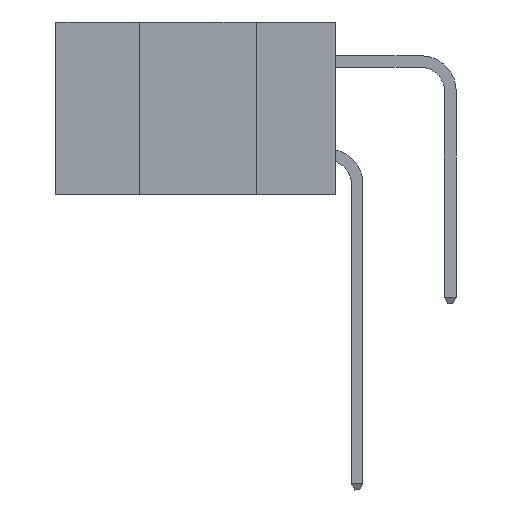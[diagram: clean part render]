
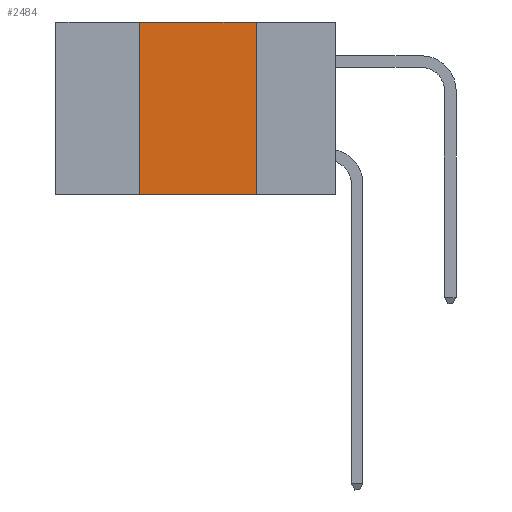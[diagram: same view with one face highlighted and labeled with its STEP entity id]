
A CAD part, left-side view. The second image highlights one B-rep face of the part: STEP entity #2484.
In plain terms, the highlighted planar face has unit normal (-1, 0, 0).
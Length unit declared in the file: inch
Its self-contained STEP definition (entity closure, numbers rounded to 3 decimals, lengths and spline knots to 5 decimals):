
#271 = ORIENTED_EDGE ( 'NONE', *, *, #18423, .F. ) ;
#292 = VECTOR ( 'NONE', #7516, 39.37008 ) ;
#970 = AXIS2_PLACEMENT_3D ( 'NONE', #7529, #13797, #14247 ) ;
#1434 = LINE ( 'NONE', #8473, #26179 ) ;
#1643 = VERTEX_POINT ( 'NONE', #16761 ) ;
#2484 = ADVANCED_FACE ( 'NONE', ( #3486 ), #12057, .F. ) ;
#2525 = VECTOR ( 'NONE', #13872, 39.37008 ) ;
#2787 = CARTESIAN_POINT ( 'NONE',  ( 0., 0.42, -0.37 ) ) ;
#3486 = FACE_OUTER_BOUND ( 'NONE', #3896, .T. ) ;
#3793 = CARTESIAN_POINT ( 'NONE',  ( 0., 0.42, 0. ) ) ;
#3896 = EDGE_LOOP ( 'NONE', ( #23246, #271, #9026, #25586 ) ) ;
#6519 = LINE ( 'NONE', #3793, #11027 ) ;
#6774 = LINE ( 'NONE', #26306, #2525 ) ;
#7516 = DIRECTION ( 'NONE',  ( 0., -1., 0. ) ) ;
#7529 = CARTESIAN_POINT ( 'NONE',  ( 0., 0.6, 0. ) ) ;
#8417 = EDGE_CURVE ( 'NONE', #19377, #11493, #6774, .T. ) ;
#8473 = CARTESIAN_POINT ( 'NONE',  ( 0., 0.17, 0. ) ) ;
#9026 = ORIENTED_EDGE ( 'NONE', *, *, #18155, .F. ) ;
#11027 = VECTOR ( 'NONE', #16083, 39.37008 ) ;
#11493 = VERTEX_POINT ( 'NONE', #21576 ) ;
#12057 = PLANE ( 'NONE',  #970 ) ;
#13797 = DIRECTION ( 'NONE',  ( 1., 0., 0. ) ) ;
#13872 = DIRECTION ( 'NONE',  ( 0., -1., 0. ) ) ;
#14247 = DIRECTION ( 'NONE',  ( 0., 0., -1. ) ) ;
#16083 = DIRECTION ( 'NONE',  ( 0., 0., 1. ) ) ;
#16761 = CARTESIAN_POINT ( 'NONE',  ( 0., 0.17, 0. ) ) ;
#17349 = EDGE_CURVE ( 'NONE', #1643, #11493, #1434, .T. ) ;
#18155 = EDGE_CURVE ( 'NONE', #19377, #22650, #6519, .T. ) ;
#18423 = EDGE_CURVE ( 'NONE', #22650, #1643, #23109, .T. ) ;
#18897 = CARTESIAN_POINT ( 'NONE',  ( 0., 0.42, 0. ) ) ;
#19138 = DIRECTION ( 'NONE',  ( 0., 0., -1. ) ) ;
#19377 = VERTEX_POINT ( 'NONE', #2787 ) ;
#21576 = CARTESIAN_POINT ( 'NONE',  ( 0., 0.17, -0.37 ) ) ;
#21626 = CARTESIAN_POINT ( 'NONE',  ( 0., 0.6, 0. ) ) ;
#22650 = VERTEX_POINT ( 'NONE', #18897 ) ;
#23109 = LINE ( 'NONE', #21626, #292 ) ;
#23246 = ORIENTED_EDGE ( 'NONE', *, *, #17349, .F. ) ;
#25586 = ORIENTED_EDGE ( 'NONE', *, *, #8417, .T. ) ;
#26179 = VECTOR ( 'NONE', #19138, 39.37008 ) ;
#26306 = CARTESIAN_POINT ( 'NONE',  ( 0., 0.6, -0.37 ) ) ;
